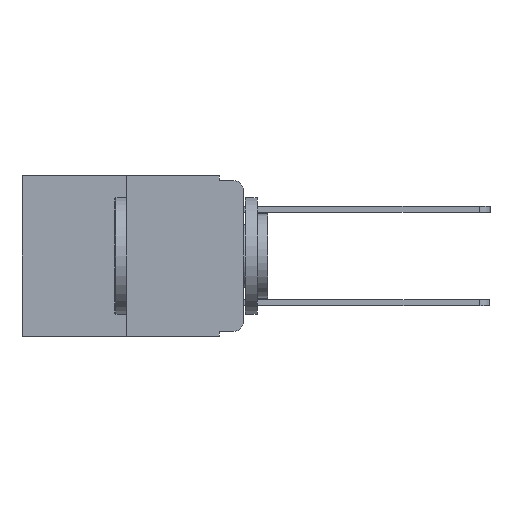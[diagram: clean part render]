
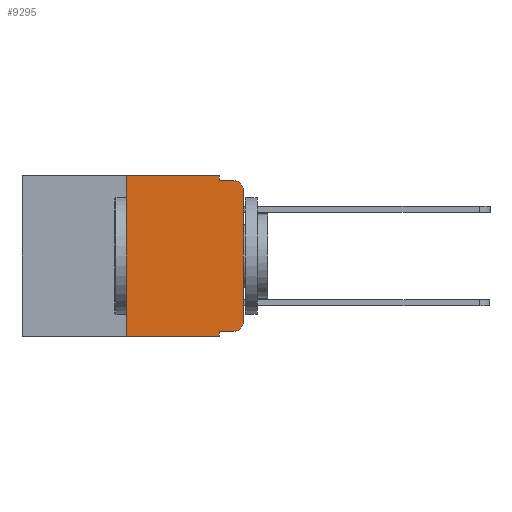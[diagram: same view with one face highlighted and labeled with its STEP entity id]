
A CAD part, left-side view. The second image highlights one B-rep face of the part: STEP entity #9295.
In plain terms, the highlighted planar face has unit normal (-1, 0, 0).
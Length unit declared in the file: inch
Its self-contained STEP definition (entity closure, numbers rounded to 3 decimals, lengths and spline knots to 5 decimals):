
#92 = VECTOR ( 'NONE', #1648, 39.37008 ) ;
#98 = AXIS2_PLACEMENT_3D ( 'NONE', #2284, #6947, #6993 ) ;
#249 = CARTESIAN_POINT ( 'NONE',  ( 0., 0.25, 0. ) ) ;
#343 = EDGE_LOOP ( 'NONE', ( #2240, #3694, #2134, #2917, #2490, #6811, #6278, #6005, #2853, #4136 ) ) ;
#447 = CARTESIAN_POINT ( 'NONE',  ( 0., 0.051, -0.343 ) ) ;
#536 = EDGE_CURVE ( 'NONE', #3760, #4011, #1536, .T. ) ;
#712 = CIRCLE ( 'NONE', #4645, 0.02 ) ;
#1070 = VECTOR ( 'NONE', #9343, 39.37008 ) ;
#1093 = EDGE_CURVE ( 'NONE', #6365, #4011, #712, .T. ) ;
#1250 = CARTESIAN_POINT ( 'NONE',  ( 0., 0., -0.313 ) ) ;
#1440 = DIRECTION ( 'NONE',  ( 0., -1., 0. ) ) ;
#1536 = LINE ( 'NONE', #4813, #9906 ) ;
#1562 = DIRECTION ( 'NONE',  ( 0., -1., 0. ) ) ;
#1620 = VECTOR ( 'NONE', #4739, 39.37008 ) ;
#1648 = DIRECTION ( 'NONE',  ( 0., 0., -1. ) ) ;
#1663 = EDGE_CURVE ( 'NONE', #6492, #6365, #8623, .T. ) ;
#2134 = ORIENTED_EDGE ( 'NONE', *, *, #536, .F. ) ;
#2240 = ORIENTED_EDGE ( 'NONE', *, *, #1663, .T. ) ;
#2284 = CARTESIAN_POINT ( 'NONE',  ( 0., 0.02, -0.313 ) ) ;
#2406 = CARTESIAN_POINT ( 'NONE',  ( 0., 0.051, -0.01 ) ) ;
#2479 = CARTESIAN_POINT ( 'NONE',  ( 0., 0.051, 0. ) ) ;
#2490 = ORIENTED_EDGE ( 'NONE', *, *, #9744, .F. ) ;
#2574 = LINE ( 'NONE', #2479, #92 ) ;
#2853 = ORIENTED_EDGE ( 'NONE', *, *, #7888, .T. ) ;
#2917 = ORIENTED_EDGE ( 'NONE', *, *, #10485, .F. ) ;
#3017 = LINE ( 'NONE', #8377, #7150 ) ;
#3208 = CARTESIAN_POINT ( 'NONE',  ( 0., 0., -0.03 ) ) ;
#3389 = VERTEX_POINT ( 'NONE', #5195 ) ;
#3472 = CARTESIAN_POINT ( 'NONE',  ( 0., 0.473, 0. ) ) ;
#3659 = CARTESIAN_POINT ( 'NONE',  ( 0., 0.02, -0.333 ) ) ;
#3694 = ORIENTED_EDGE ( 'NONE', *, *, #1093, .T. ) ;
#3760 = VERTEX_POINT ( 'NONE', #2406 ) ;
#4011 = VERTEX_POINT ( 'NONE', #4733 ) ;
#4136 = ORIENTED_EDGE ( 'NONE', *, *, #7375, .T. ) ;
#4245 = VECTOR ( 'NONE', #1562, 39.37008 ) ;
#4256 = FACE_OUTER_BOUND ( 'NONE', #343, .T. ) ;
#4290 = DIRECTION ( 'NONE',  ( 0., 0., -1. ) ) ;
#4529 = LINE ( 'NONE', #6507, #4245 ) ;
#4635 = CARTESIAN_POINT ( 'NONE',  ( 0., 0.25, 0. ) ) ;
#4645 = AXIS2_PLACEMENT_3D ( 'NONE', #7971, #5832, #9081 ) ;
#4694 = CARTESIAN_POINT ( 'NONE',  ( 0., 0.051, -0.333 ) ) ;
#4733 = CARTESIAN_POINT ( 'NONE',  ( 0., 0.02, -0.01 ) ) ;
#4739 = DIRECTION ( 'NONE',  ( 0., -1., 0. ) ) ;
#4761 = EDGE_CURVE ( 'NONE', #8930, #6874, #5481, .T. ) ;
#4813 = CARTESIAN_POINT ( 'NONE',  ( 0., 0.051, -0.01 ) ) ;
#5195 = CARTESIAN_POINT ( 'NONE',  ( 0., 0.051, 0. ) ) ;
#5344 = AXIS2_PLACEMENT_3D ( 'NONE', #3472, #9113, #4290 ) ;
#5481 = LINE ( 'NONE', #8330, #1070 ) ;
#5832 = DIRECTION ( 'NONE',  ( -1., 0., 0. ) ) ;
#6005 = ORIENTED_EDGE ( 'NONE', *, *, #8401, .F. ) ;
#6278 = ORIENTED_EDGE ( 'NONE', *, *, #4761, .T. ) ;
#6365 = VERTEX_POINT ( 'NONE', #3208 ) ;
#6470 = DIRECTION ( 'NONE',  ( 0., 0., 1. ) ) ;
#6492 = VERTEX_POINT ( 'NONE', #1250 ) ;
#6507 = CARTESIAN_POINT ( 'NONE',  ( 0., 0.473, 0. ) ) ;
#6522 = CARTESIAN_POINT ( 'NONE',  ( 0., 0., 0. ) ) ;
#6542 = VECTOR ( 'NONE', #6470, 39.37008 ) ;
#6756 = VERTEX_POINT ( 'NONE', #249 ) ;
#6811 = ORIENTED_EDGE ( 'NONE', *, *, #8941, .F. ) ;
#6874 = VERTEX_POINT ( 'NONE', #447 ) ;
#6947 = DIRECTION ( 'NONE',  ( -1., 0., 0. ) ) ;
#6993 = DIRECTION ( 'NONE',  ( 0., 0., -1. ) ) ;
#7150 = VECTOR ( 'NONE', #7415, 39.37008 ) ;
#7375 = EDGE_CURVE ( 'NONE', #8313, #6492, #8981, .T. ) ;
#7415 = DIRECTION ( 'NONE',  ( 0., 0., -1. ) ) ;
#7666 = VERTEX_POINT ( 'NONE', #8482 ) ;
#7855 = LINE ( 'NONE', #4635, #9955 ) ;
#7888 = EDGE_CURVE ( 'NONE', #7666, #8313, #8122, .T. ) ;
#7971 = CARTESIAN_POINT ( 'NONE',  ( 0., 0.02, -0.03 ) ) ;
#8122 = LINE ( 'NONE', #4694, #1620 ) ;
#8313 = VERTEX_POINT ( 'NONE', #3659 ) ;
#8328 = PLANE ( 'NONE',  #5344 ) ;
#8330 = CARTESIAN_POINT ( 'NONE',  ( 0., 0.473, -0.343 ) ) ;
#8377 = CARTESIAN_POINT ( 'NONE',  ( 0., 0.051, 0. ) ) ;
#8401 = EDGE_CURVE ( 'NONE', #7666, #6874, #3017, .T. ) ;
#8482 = CARTESIAN_POINT ( 'NONE',  ( 0., 0.051, -0.333 ) ) ;
#8623 = LINE ( 'NONE', #6522, #6542 ) ;
#8930 = VERTEX_POINT ( 'NONE', #10194 ) ;
#8941 = EDGE_CURVE ( 'NONE', #8930, #6756, #7855, .T. ) ;
#8981 = CIRCLE ( 'NONE', #98, 0.02 ) ;
#9081 = DIRECTION ( 'NONE',  ( 0., 0., -1. ) ) ;
#9113 = DIRECTION ( 'NONE',  ( 1., 0., 0. ) ) ;
#9295 = ADVANCED_FACE ( 'NONE', ( #4256 ), #8328, .F. ) ;
#9343 = DIRECTION ( 'NONE',  ( 0., -1., 0. ) ) ;
#9744 = EDGE_CURVE ( 'NONE', #6756, #3389, #4529, .T. ) ;
#9906 = VECTOR ( 'NONE', #1440, 39.37008 ) ;
#9955 = VECTOR ( 'NONE', #10219, 39.37008 ) ;
#10194 = CARTESIAN_POINT ( 'NONE',  ( 0., 0.25, -0.343 ) ) ;
#10219 = DIRECTION ( 'NONE',  ( 0., 0., 1. ) ) ;
#10485 = EDGE_CURVE ( 'NONE', #3389, #3760, #2574, .T. ) ;
